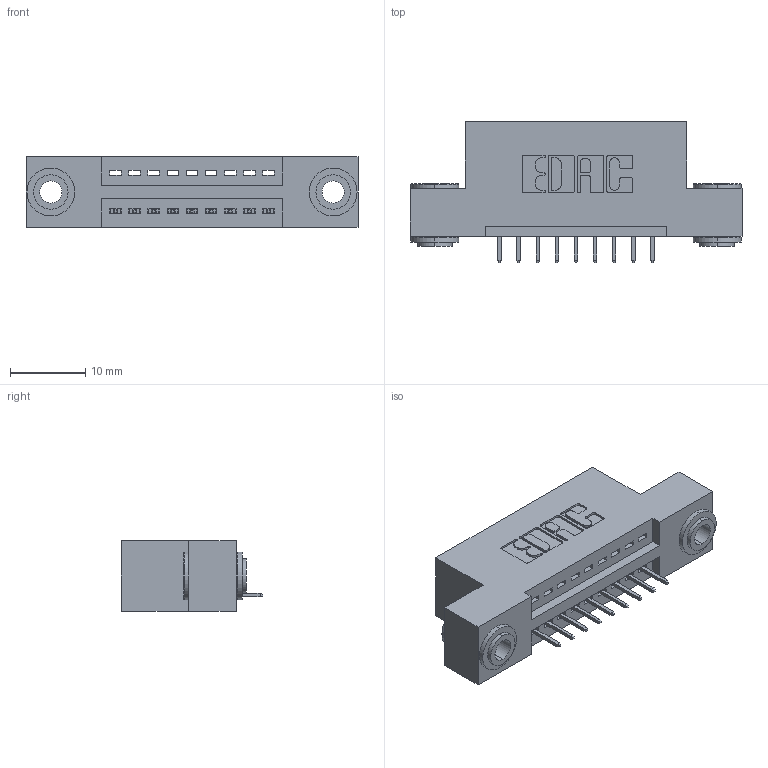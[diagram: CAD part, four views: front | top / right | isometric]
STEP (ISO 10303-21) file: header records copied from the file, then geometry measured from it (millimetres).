
FILE_DESCRIPTION (( 'STEP AP203' ), '1' );
FILE_NAME ('845-009-525-103.STEP', '2020-09-22T15:08:37', ( '' ), ( '' ), 'SwSTEP 2.0', 'SolidWorks 2020', '' );
FILE_SCHEMA (( 'CONFIG_CONTROL_DESIGN' ));
Length unit declared in the file: inch
Products named in the file (4): 345-250-002_345-250-002-102; 845 Part_Flush Mounting Lugs - 0.156 Dia-TH; 345-292-001_345-293-125; 845-009-525-103
Assembly tree (12 placements, depth 2):
  845-009-525-103
    845 Part_Flush Mounting Lugs - 0.156 Dia-TH
    345-292-001_345-293-125  x9
    345-250-002_345-250-002-102  x2
Bounding box: 44.07 x 18.72 x 9.4 mm (x, y, z)
Volume: 3898 mm3; surface area: 4823.6 mm2
Topology: 12 solids, 12 shells, 722 faces, 2037 edges, 1318 vertices
Faces by surface type: plane 504, cylinder 210, cone 8
Entity records: 11940 total; most frequent: CARTESIAN_POINT 2046, ORIENTED_EDGE 1982, DIRECTION 1867, EDGE_CURVE 991, VECTOR 803, LINE 803, VERTEX_POINT 654, AXIS2_PLACEMENT_3D 532
